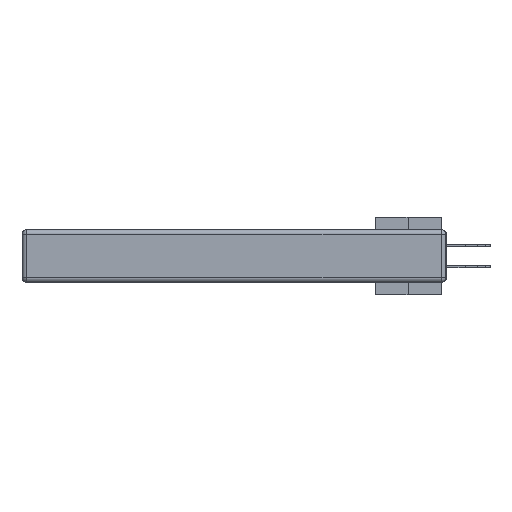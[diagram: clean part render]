
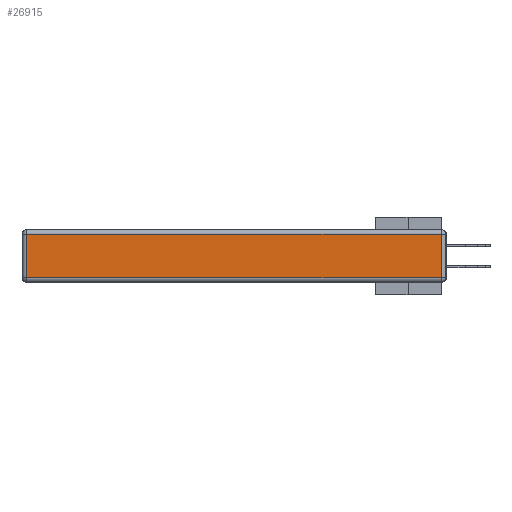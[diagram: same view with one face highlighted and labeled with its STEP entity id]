
A CAD part, left-side view. The second image highlights one B-rep face of the part: STEP entity #26915.
In plain terms, the highlighted planar face has unit normal (-1, 0, 0).
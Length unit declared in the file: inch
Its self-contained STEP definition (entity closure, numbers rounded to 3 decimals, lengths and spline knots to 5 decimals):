
#684 = CARTESIAN_POINT ( 'NONE',  ( 0., 0.03, -0.03 ) ) ;
#933 = DIRECTION ( 'NONE',  ( 0., 1., 0. ) ) ;
#939 = CARTESIAN_POINT ( 'NONE',  ( 0., 0.03, -0.343 ) ) ;
#1676 = VECTOR ( 'NONE', #933, 39.37008 ) ;
#3531 = FACE_OUTER_BOUND ( 'NONE', #32485, .T. ) ;
#4158 = VERTEX_POINT ( 'NONE', #9218 ) ;
#4221 = DIRECTION ( 'NONE',  ( 0., 0., 1. ) ) ;
#4592 = AXIS2_PLACEMENT_3D ( 'NONE', #30601, #22100, #7228 ) ;
#4635 = EDGE_CURVE ( 'NONE', #16847, #4158, #15852, .T. ) ;
#4709 = CARTESIAN_POINT ( 'NONE',  ( 0., 2.72, -0.313 ) ) ;
#4953 = DIRECTION ( 'NONE',  ( 0., 0., -1. ) ) ;
#6578 = LINE ( 'NONE', #19191, #9311 ) ;
#7228 = DIRECTION ( 'NONE',  ( 0., 0., 1. ) ) ;
#7636 = ORIENTED_EDGE ( 'NONE', *, *, #24573, .T. ) ;
#8175 = LINE ( 'NONE', #939, #28649 ) ;
#9218 = CARTESIAN_POINT ( 'NONE',  ( 0., 2.72, -0.03 ) ) ;
#9311 = VECTOR ( 'NONE', #4953, 39.37008 ) ;
#9640 = ORIENTED_EDGE ( 'NONE', *, *, #36693, .T. ) ;
#10322 = ORIENTED_EDGE ( 'NONE', *, *, #4635, .T. ) ;
#10477 = ORIENTED_EDGE ( 'NONE', *, *, #37045, .T. ) ;
#12478 = VECTOR ( 'NONE', #18513, 39.37008 ) ;
#15852 = LINE ( 'NONE', #18622, #1676 ) ;
#16211 = VERTEX_POINT ( 'NONE', #25091 ) ;
#16847 = VERTEX_POINT ( 'NONE', #684 ) ;
#18513 = DIRECTION ( 'NONE',  ( 0., -1., 0. ) ) ;
#18622 = CARTESIAN_POINT ( 'NONE',  ( 0., 2.75, -0.03 ) ) ;
#19191 = CARTESIAN_POINT ( 'NONE',  ( 0., 2.72, -0.343 ) ) ;
#22100 = DIRECTION ( 'NONE',  ( -1., 0., 0. ) ) ;
#24259 = PLANE ( 'NONE',  #4592 ) ;
#24573 = EDGE_CURVE ( 'NONE', #16211, #16847, #8175, .T. ) ;
#25091 = CARTESIAN_POINT ( 'NONE',  ( 0., 0.03, -0.313 ) ) ;
#26915 = ADVANCED_FACE ( 'NONE', ( #3531 ), #24259, .T. ) ;
#28649 = VECTOR ( 'NONE', #4221, 39.37008 ) ;
#30601 = CARTESIAN_POINT ( 'NONE',  ( 0., 0., -0.343 ) ) ;
#32001 = VERTEX_POINT ( 'NONE', #4709 ) ;
#32485 = EDGE_LOOP ( 'NONE', ( #10477, #7636, #10322, #9640 ) ) ;
#33006 = CARTESIAN_POINT ( 'NONE',  ( 0., 0., -0.313 ) ) ;
#36693 = EDGE_CURVE ( 'NONE', #4158, #32001, #6578, .T. ) ;
#37045 = EDGE_CURVE ( 'NONE', #32001, #16211, #37077, .T. ) ;
#37077 = LINE ( 'NONE', #33006, #12478 ) ;
